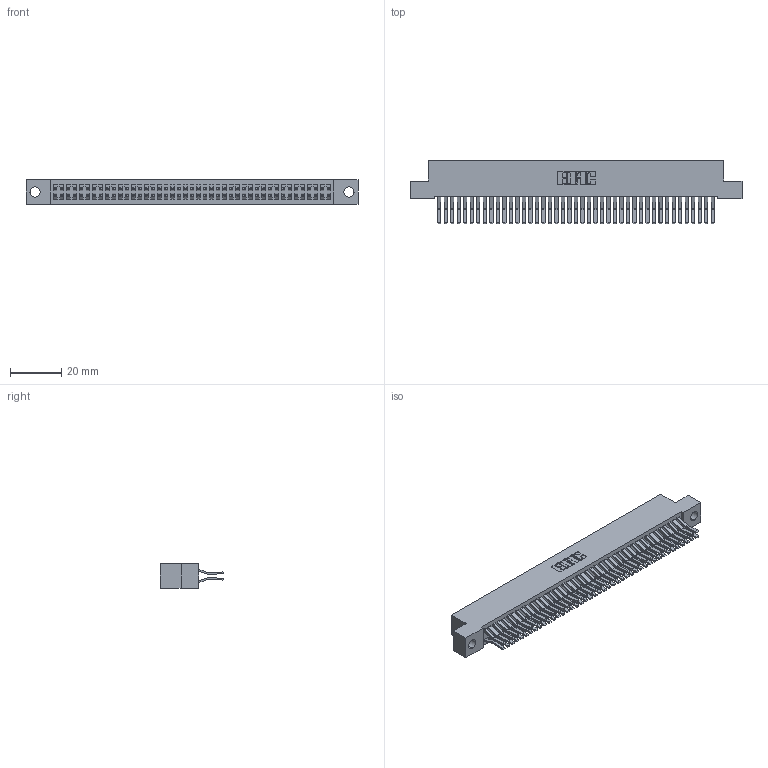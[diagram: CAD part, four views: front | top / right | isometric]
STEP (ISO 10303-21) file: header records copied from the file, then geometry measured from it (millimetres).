
FILE_DESCRIPTION (( 'STEP AP203' ), '1' );
FILE_NAME ('392-086-560-204.STEP', '2019-10-09T16:33:05', ( '' ), ( '' ), 'SwSTEP 2.0', 'SolidWorks 2016', '' );
FILE_SCHEMA (( 'CONFIG_CONTROL_DESIGN' ));
Length unit declared in the file: inch
Products named in the file (3): 345-292-001_560 Tail; 392-086-560-204; 342 Part_.156 TH
Assembly tree (87 placements, depth 2):
  392-086-560-204
    342 Part_.156 TH
    345-292-001_560 Tail  x86
Bounding box: 129.54 x 24.78 x 9.4 mm (x, y, z)
Volume: 12121.5 mm3; surface area: 20933.4 mm2
Topology: 87 solids, 87 shells, 4754 faces, 14145 edges, 9314 vertices
Faces by surface type: plane 3162, cylinder 1592
Entity records: 27493 total; most frequent: CARTESIAN_POINT 4554, ORIENTED_EDGE 4490, DIRECTION 3893, EDGE_CURVE 2245, VECTOR 2113, LINE 2113, VERTEX_POINT 1494, AXIS2_PLACEMENT_3D 890
